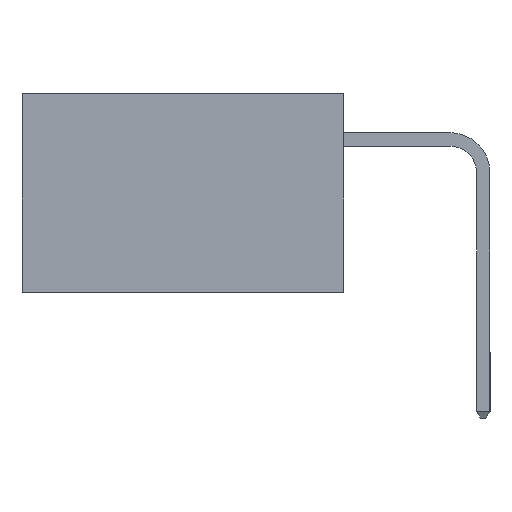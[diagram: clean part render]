
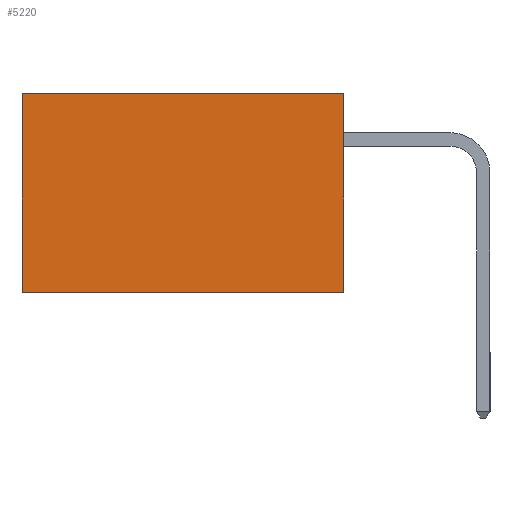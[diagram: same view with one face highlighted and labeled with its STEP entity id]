
A CAD part, left-side view. The second image highlights one B-rep face of the part: STEP entity #5220.
In plain terms, the highlighted planar face has unit normal (-1, 0, 0).
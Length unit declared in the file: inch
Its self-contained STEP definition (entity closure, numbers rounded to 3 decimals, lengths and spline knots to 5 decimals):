
#251 = EDGE_CURVE ( 'NONE', #6772, #966, #8142, .T. ) ;
#966 = VERTEX_POINT ( 'NONE', #9234 ) ;
#1046 = DIRECTION ( 'NONE',  ( 0., 1., 0. ) ) ;
#1890 = VECTOR ( 'NONE', #14745, 39.37008 ) ;
#2092 = VECTOR ( 'NONE', #6754, 39.37008 ) ;
#2211 = ORIENTED_EDGE ( 'NONE', *, *, #251, .T. ) ;
#2522 = DIRECTION ( 'NONE',  ( 0., 0., -1. ) ) ;
#2869 = EDGE_CURVE ( 'NONE', #966, #4783, #12189, .T. ) ;
#3181 = AXIS2_PLACEMENT_3D ( 'NONE', #5214, #3374, #10432 ) ;
#3204 = PLANE ( 'NONE',  #3181 ) ;
#3374 = DIRECTION ( 'NONE',  ( 1., 0., 0. ) ) ;
#4265 = CARTESIAN_POINT ( 'NONE',  ( 0.298, 0., 0. ) ) ;
#4783 = VERTEX_POINT ( 'NONE', #11925 ) ;
#4967 = LINE ( 'NONE', #5365, #1890 ) ;
#5214 = CARTESIAN_POINT ( 'NONE',  ( 0.298, 0., 0. ) ) ;
#5220 = ADVANCED_FACE ( 'NONE', ( #6857 ), #3204, .F. ) ;
#5365 = CARTESIAN_POINT ( 'NONE',  ( 0.298, 0., -0.37 ) ) ;
#5706 = ORIENTED_EDGE ( 'NONE', *, *, #2869, .T. ) ;
#6754 = DIRECTION ( 'NONE',  ( 0., 0., -1. ) ) ;
#6772 = VERTEX_POINT ( 'NONE', #6946 ) ;
#6785 = EDGE_LOOP ( 'NONE', ( #5706, #12359, #7062, #2211 ) ) ;
#6857 = FACE_OUTER_BOUND ( 'NONE', #6785, .T. ) ;
#6946 = CARTESIAN_POINT ( 'NONE',  ( 0.298, 0., 0. ) ) ;
#7062 = ORIENTED_EDGE ( 'NONE', *, *, #10016, .F. ) ;
#7998 = CARTESIAN_POINT ( 'NONE',  ( 0.298, 0., 0. ) ) ;
#8142 = LINE ( 'NONE', #7998, #13438 ) ;
#9234 = CARTESIAN_POINT ( 'NONE',  ( 0.298, 0.6, 0. ) ) ;
#10016 = EDGE_CURVE ( 'NONE', #6772, #14647, #14471, .T. ) ;
#10432 = DIRECTION ( 'NONE',  ( 0., 0., -1. ) ) ;
#10517 = CARTESIAN_POINT ( 'NONE',  ( 0.298, 0., -0.37 ) ) ;
#10695 = EDGE_CURVE ( 'NONE', #14647, #4783, #4967, .T. ) ;
#10744 = CARTESIAN_POINT ( 'NONE',  ( 0.298, 0.6, 0. ) ) ;
#11280 = VECTOR ( 'NONE', #2522, 39.37008 ) ;
#11925 = CARTESIAN_POINT ( 'NONE',  ( 0.298, 0.6, -0.37 ) ) ;
#12189 = LINE ( 'NONE', #10744, #11280 ) ;
#12359 = ORIENTED_EDGE ( 'NONE', *, *, #10695, .F. ) ;
#13438 = VECTOR ( 'NONE', #1046, 39.37008 ) ;
#14471 = LINE ( 'NONE', #4265, #2092 ) ;
#14647 = VERTEX_POINT ( 'NONE', #10517 ) ;
#14745 = DIRECTION ( 'NONE',  ( 0., 1., 0. ) ) ;
